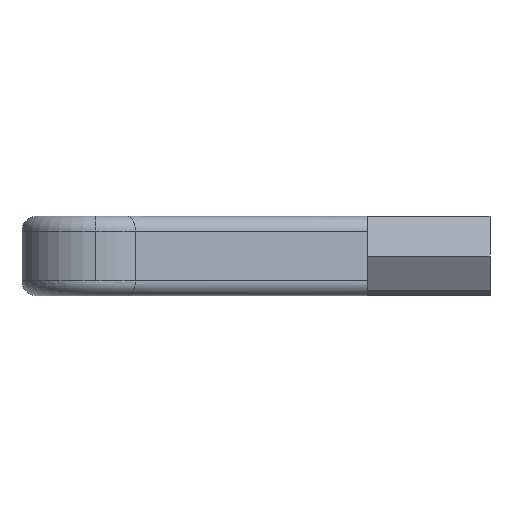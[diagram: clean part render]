
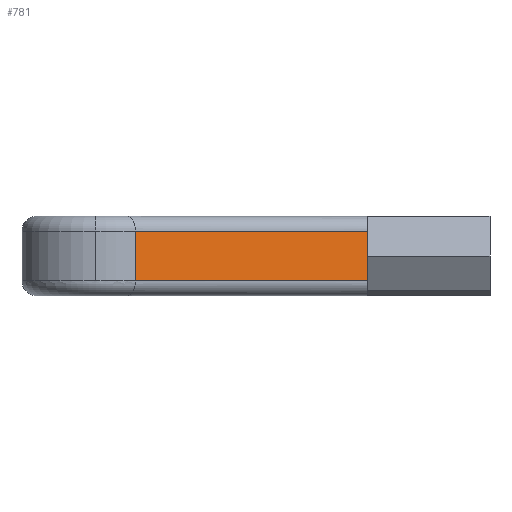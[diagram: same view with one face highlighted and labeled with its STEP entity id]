
A CAD part, left-side view. The second image highlights one B-rep face of the part: STEP entity #781.
In plain terms, the highlighted planar face has unit normal (-0.844, -0.536, 0).
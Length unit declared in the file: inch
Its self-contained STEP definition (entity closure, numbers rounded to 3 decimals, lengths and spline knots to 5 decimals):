
#227 = CARTESIAN_POINT ( 'NONE',  ( -0.21223, -0.17, -0.08455 ) ) ;
#289 = CARTESIAN_POINT ( 'NONE',  ( -0.21223, -0.17, -1.75948 ) ) ;
#419 = VERTEX_POINT ( 'NONE', #581 ) ;
#534 = EDGE_CURVE ( 'NONE', #1059, #700, #693, .T. ) ;
#541 = EDGE_LOOP ( 'NONE', ( #628, #1893, #1395, #1874 ) ) ;
#581 = CARTESIAN_POINT ( 'NONE',  ( -0.21223, -0.17, 0.08455 ) ) ;
#628 = ORIENTED_EDGE ( 'NONE', *, *, #534, .F. ) ;
#640 = VECTOR ( 'NONE', #933, 39.37008 ) ;
#689 = DIRECTION ( 'NONE',  ( -0.536, 0.844, 0. ) ) ;
#693 = LINE ( 'NONE', #1162, #1886 ) ;
#700 = VERTEX_POINT ( 'NONE', #1194 ) ;
#781 = ADVANCED_FACE ( 'NONE', ( #1580 ), #1228, .T. ) ;
#798 = CARTESIAN_POINT ( 'NONE',  ( -0.71108, 0.61604, -0.08455 ) ) ;
#933 = DIRECTION ( 'NONE',  ( 0.536, -0.844, 0. ) ) ;
#940 = CARTESIAN_POINT ( 'NONE',  ( -0.21223, -0.17, -0.08455 ) ) ;
#1059 = VERTEX_POINT ( 'NONE', #798 ) ;
#1147 = EDGE_CURVE ( 'NONE', #1870, #419, #1785, .T. ) ;
#1162 = CARTESIAN_POINT ( 'NONE',  ( -0.71108, 0.61604, -1.75948 ) ) ;
#1194 = CARTESIAN_POINT ( 'NONE',  ( -0.71108, 0.61604, 0.08455 ) ) ;
#1226 = CARTESIAN_POINT ( 'NONE',  ( -0.21223, -0.17, -1.75948 ) ) ;
#1228 = PLANE ( 'NONE',  #1974 ) ;
#1251 = EDGE_CURVE ( 'NONE', #1059, #1870, #1812, .T. ) ;
#1325 = DIRECTION ( 'NONE',  ( 0., 0., 1. ) ) ;
#1358 = VECTOR ( 'NONE', #689, 39.37008 ) ;
#1361 = VECTOR ( 'NONE', #1381, 39.37008 ) ;
#1381 = DIRECTION ( 'NONE',  ( 0., 0., 1. ) ) ;
#1395 = ORIENTED_EDGE ( 'NONE', *, *, #1147, .T. ) ;
#1477 = EDGE_CURVE ( 'NONE', #419, #700, #1783, .T. ) ;
#1580 = FACE_OUTER_BOUND ( 'NONE', #541, .T. ) ;
#1639 = CARTESIAN_POINT ( 'NONE',  ( -0.71108, 0.61604, 0.08455 ) ) ;
#1694 = DIRECTION ( 'NONE',  ( -0.844, -0.536, 0. ) ) ;
#1713 = DIRECTION ( 'NONE',  ( 0.536, -0.844, 0. ) ) ;
#1783 = LINE ( 'NONE', #1639, #1358 ) ;
#1785 = LINE ( 'NONE', #1226, #1361 ) ;
#1812 = LINE ( 'NONE', #940, #640 ) ;
#1870 = VERTEX_POINT ( 'NONE', #227 ) ;
#1874 = ORIENTED_EDGE ( 'NONE', *, *, #1477, .T. ) ;
#1886 = VECTOR ( 'NONE', #1325, 39.37008 ) ;
#1893 = ORIENTED_EDGE ( 'NONE', *, *, #1251, .T. ) ;
#1974 = AXIS2_PLACEMENT_3D ( 'NONE', #289, #1694, #1713 ) ;
